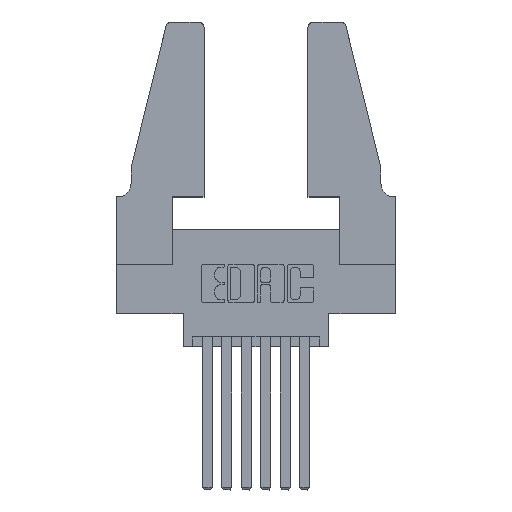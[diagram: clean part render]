
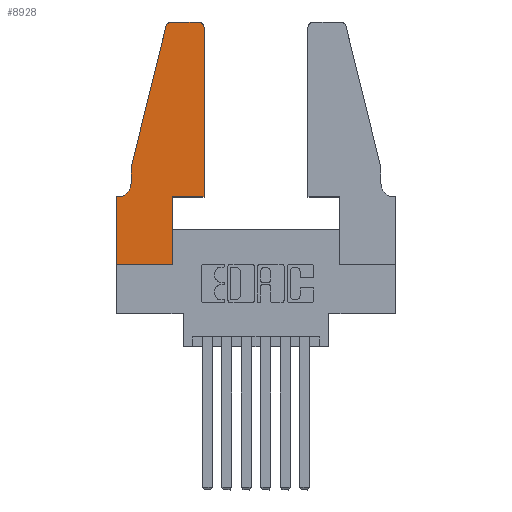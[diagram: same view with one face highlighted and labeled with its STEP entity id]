
A CAD part, top view. The second image highlights one B-rep face of the part: STEP entity #8928.
In plain terms, the highlighted planar face has unit normal (0, 0, 1).
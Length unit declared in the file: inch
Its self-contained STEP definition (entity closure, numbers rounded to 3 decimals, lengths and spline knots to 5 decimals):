
#94 = CARTESIAN_POINT ( 'NONE',  ( 0.4505, 1.22, 0.37 ) ) ;
#98 = EDGE_LOOP ( 'NONE', ( #334, #7903, #1194, #1309, #2533, #1731, #6968, #2171, #5053, #9138, #5470, #3042 ) ) ;
#251 = CARTESIAN_POINT ( 'NONE',  ( 0., 0.35, 0.37 ) ) ;
#334 = ORIENTED_EDGE ( 'NONE', *, *, #10209, .T. ) ;
#384 = LINE ( 'NONE', #9791, #7331 ) ;
#718 = VERTEX_POINT ( 'NONE', #94 ) ;
#879 = VECTOR ( 'NONE', #7242, 39.37008 ) ;
#919 = EDGE_CURVE ( 'NONE', #4067, #4346, #5650, .T. ) ;
#1194 = ORIENTED_EDGE ( 'NONE', *, *, #919, .T. ) ;
#1245 = DIRECTION ( 'NONE',  ( 1., 0., 0. ) ) ;
#1308 = DIRECTION ( 'NONE',  ( -1., 0., 0. ) ) ;
#1309 = ORIENTED_EDGE ( 'NONE', *, *, #2555, .T. ) ;
#1449 = VERTEX_POINT ( 'NONE', #9787 ) ;
#1731 = ORIENTED_EDGE ( 'NONE', *, *, #10765, .T. ) ;
#1752 = CARTESIAN_POINT ( 'NONE',  ( 0., 0.35, 0.37 ) ) ;
#1787 = AXIS2_PLACEMENT_3D ( 'NONE', #251, #6574, #1245 ) ;
#1866 = CIRCLE ( 'NONE', #6950, 0.03 ) ;
#2076 = EDGE_CURVE ( 'NONE', #718, #10306, #2193, .T. ) ;
#2108 = CARTESIAN_POINT ( 'NONE',  ( 0.4505, 0.35, 0.37 ) ) ;
#2155 = FACE_OUTER_BOUND ( 'NONE', #98, .T. ) ;
#2171 = ORIENTED_EDGE ( 'NONE', *, *, #4442, .T. ) ;
#2193 = CIRCLE ( 'NONE', #6473, 0.03 ) ;
#2209 = CARTESIAN_POINT ( 'NONE',  ( 0., 0., 0.37 ) ) ;
#2217 = CARTESIAN_POINT ( 'NONE',  ( 0.2605, 1.25, 0.37 ) ) ;
#2432 = DIRECTION ( 'NONE',  ( 0., -1., 0. ) ) ;
#2500 = LINE ( 'NONE', #7033, #11654 ) ;
#2533 = ORIENTED_EDGE ( 'NONE', *, *, #10505, .T. ) ;
#2555 = EDGE_CURVE ( 'NONE', #4346, #7466, #4536, .T. ) ;
#2557 = CARTESIAN_POINT ( 'NONE',  ( 0.284, 1.22, 0.37 ) ) ;
#2666 = DIRECTION ( 'NONE',  ( 0., 1., 0. ) ) ;
#2682 = DIRECTION ( 'NONE',  ( -1., 0., 0. ) ) ;
#2729 = CARTESIAN_POINT ( 'NONE',  ( 0.0755, 0.42, 0.37 ) ) ;
#2907 = LINE ( 'NONE', #7444, #9700 ) ;
#3042 = ORIENTED_EDGE ( 'NONE', *, *, #2076, .T. ) ;
#3474 = DIRECTION ( 'NONE',  ( 1., 0., 0. ) ) ;
#3515 = CARTESIAN_POINT ( 'NONE',  ( 0.0055, 0.42, 0.37 ) ) ;
#4067 = VERTEX_POINT ( 'NONE', #8057 ) ;
#4346 = VERTEX_POINT ( 'NONE', #7039 ) ;
#4380 = DIRECTION ( 'NONE',  ( -1., 0., 0. ) ) ;
#4442 = EDGE_CURVE ( 'NONE', #10977, #7443, #6757, .T. ) ;
#4458 = VECTOR ( 'NONE', #5751, 39.37008 ) ;
#4466 = CARTESIAN_POINT ( 'NONE',  ( 0.2865, 0., 0.37 ) ) ;
#4536 = LINE ( 'NONE', #10793, #8994 ) ;
#4812 = PLANE ( 'NONE',  #1787 ) ;
#4947 = DIRECTION ( 'NONE',  ( 1., 0., 0. ) ) ;
#4976 = DIRECTION ( 'NONE',  ( 0., 0., 1. ) ) ;
#5007 = CARTESIAN_POINT ( 'NONE',  ( 0.4205, 1.22, 0.37 ) ) ;
#5009 = VECTOR ( 'NONE', #7073, 39.37008 ) ;
#5053 = ORIENTED_EDGE ( 'NONE', *, *, #5068, .T. ) ;
#5068 = EDGE_CURVE ( 'NONE', #7443, #9760, #2500, .T. ) ;
#5303 = CARTESIAN_POINT ( 'NONE',  ( 0., 0., 0.37 ) ) ;
#5470 = ORIENTED_EDGE ( 'NONE', *, *, #10087, .T. ) ;
#5650 = LINE ( 'NONE', #10620, #879 ) ;
#5751 = DIRECTION ( 'NONE',  ( 1., 0., 0. ) ) ;
#6084 = CARTESIAN_POINT ( 'NONE',  ( 0.0055, 0.35, 0.37 ) ) ;
#6304 = VERTEX_POINT ( 'NONE', #9043 ) ;
#6473 = AXIS2_PLACEMENT_3D ( 'NONE', #5007, #4976, #4947 ) ;
#6574 = DIRECTION ( 'NONE',  ( 0., 0., 1. ) ) ;
#6757 = LINE ( 'NONE', #2209, #4458 ) ;
#6950 = AXIS2_PLACEMENT_3D ( 'NONE', #2557, #8743, #3474 ) ;
#6968 = ORIENTED_EDGE ( 'NONE', *, *, #9309, .T. ) ;
#7033 = CARTESIAN_POINT ( 'NONE',  ( 0.2865, 0.35, 0.37 ) ) ;
#7039 = CARTESIAN_POINT ( 'NONE',  ( 0.0755, 0.5, 0.37 ) ) ;
#7073 = DIRECTION ( 'NONE',  ( 0., -1., 0. ) ) ;
#7242 = DIRECTION ( 'NONE',  ( -0.239, -0.971, 0. ) ) ;
#7331 = VECTOR ( 'NONE', #2682, 39.37008 ) ;
#7371 = VECTOR ( 'NONE', #1308, 39.37008 ) ;
#7379 = VERTEX_POINT ( 'NONE', #6084 ) ;
#7380 = CARTESIAN_POINT ( 'NONE',  ( 0., 0., 0.37 ) ) ;
#7399 = LINE ( 'NONE', #2108, #11173 ) ;
#7443 = VERTEX_POINT ( 'NONE', #4466 ) ;
#7444 = CARTESIAN_POINT ( 'NONE',  ( 0.4505, 0.35, 0.37 ) ) ;
#7449 = AXIS2_PLACEMENT_3D ( 'NONE', #3515, #9717, #4380 ) ;
#7466 = VERTEX_POINT ( 'NONE', #2729 ) ;
#7652 = LINE ( 'NONE', #2217, #7371 ) ;
#7669 = LINE ( 'NONE', #5303, #5009 ) ;
#7903 = ORIENTED_EDGE ( 'NONE', *, *, #8517, .T. ) ;
#8057 = CARTESIAN_POINT ( 'NONE',  ( 0.25487, 1.22718, 0.37 ) ) ;
#8517 = EDGE_CURVE ( 'NONE', #6304, #4067, #1866, .T. ) ;
#8743 = DIRECTION ( 'NONE',  ( 0., 0., 1. ) ) ;
#8928 = ADVANCED_FACE ( 'NONE', ( #2155 ), #4812, .T. ) ;
#8994 = VECTOR ( 'NONE', #2432, 39.37008 ) ;
#9043 = CARTESIAN_POINT ( 'NONE',  ( 0.284, 1.25, 0.37 ) ) ;
#9138 = ORIENTED_EDGE ( 'NONE', *, *, #11607, .T. ) ;
#9309 = EDGE_CURVE ( 'NONE', #11341, #10977, #7669, .T. ) ;
#9647 = CARTESIAN_POINT ( 'NONE',  ( 0.2865, 0.35, 0.37 ) ) ;
#9700 = VECTOR ( 'NONE', #10184, 39.37008 ) ;
#9717 = DIRECTION ( 'NONE',  ( 0., 0., -1. ) ) ;
#9760 = VERTEX_POINT ( 'NONE', #9647 ) ;
#9787 = CARTESIAN_POINT ( 'NONE',  ( 0.4505, 0.35, 0.37 ) ) ;
#9791 = CARTESIAN_POINT ( 'NONE',  ( 0.0755, 0.35, 0.37 ) ) ;
#10087 = EDGE_CURVE ( 'NONE', #1449, #718, #7399, .T. ) ;
#10131 = DIRECTION ( 'NONE',  ( 0., 1., 0. ) ) ;
#10184 = DIRECTION ( 'NONE',  ( 1., 0., 0. ) ) ;
#10209 = EDGE_CURVE ( 'NONE', #10306, #6304, #7652, .T. ) ;
#10306 = VERTEX_POINT ( 'NONE', #11232 ) ;
#10505 = EDGE_CURVE ( 'NONE', #7466, #7379, #10724, .T. ) ;
#10620 = CARTESIAN_POINT ( 'NONE',  ( 0.0755, 0.5, 0.37 ) ) ;
#10724 = CIRCLE ( 'NONE', #7449, 0.07 ) ;
#10765 = EDGE_CURVE ( 'NONE', #7379, #11341, #384, .T. ) ;
#10793 = CARTESIAN_POINT ( 'NONE',  ( 0.0755, 0.5, 0.37 ) ) ;
#10977 = VERTEX_POINT ( 'NONE', #7380 ) ;
#11173 = VECTOR ( 'NONE', #10131, 39.37008 ) ;
#11232 = CARTESIAN_POINT ( 'NONE',  ( 0.4205, 1.25, 0.37 ) ) ;
#11341 = VERTEX_POINT ( 'NONE', #1752 ) ;
#11607 = EDGE_CURVE ( 'NONE', #9760, #1449, #2907, .T. ) ;
#11654 = VECTOR ( 'NONE', #2666, 39.37008 ) ;
